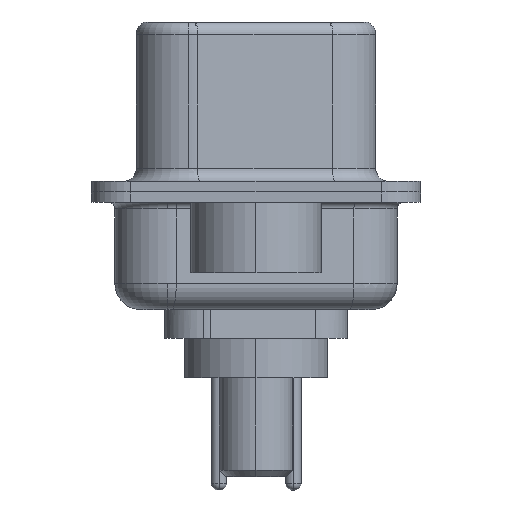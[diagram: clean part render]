
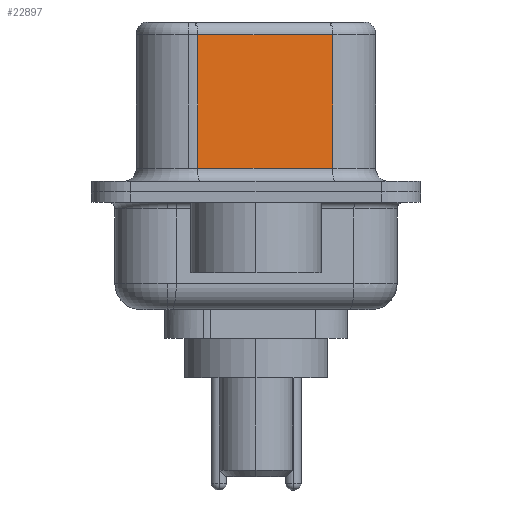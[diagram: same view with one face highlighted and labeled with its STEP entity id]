
A CAD part, left-side view. The second image highlights one B-rep face of the part: STEP entity #22897.
In plain terms, the highlighted planar face has unit normal (-0.985, -0.174, 0).
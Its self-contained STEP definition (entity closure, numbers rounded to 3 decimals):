
#64 = VERTEX_POINT ( 'NONE', #10627 ) ;
#67 = EDGE_CURVE ( 'NONE', #1462, #18568, #2267, .T. ) ;
#1438 = ORIENTED_EDGE ( 'NONE', *, *, #24610, .T. ) ;
#1462 = VERTEX_POINT ( 'NONE', #10594 ) ;
#1481 = CARTESIAN_POINT ( 'NONE',  ( 4.58, -2.927, 6.52 ) ) ;
#2267 = LINE ( 'NONE', #23802, #22901 ) ;
#2606 = VECTOR ( 'NONE', #9799, 1000. ) ;
#3443 = DIRECTION ( 'NONE',  ( 0.985, 0.174, 0. ) ) ;
#3706 = VERTEX_POINT ( 'NONE', #5893 ) ;
#5893 = CARTESIAN_POINT ( 'NONE',  ( 3.67, 2.233, 0.9 ) ) ;
#5898 = LINE ( 'NONE', #21423, #21189 ) ;
#6549 = FACE_OUTER_BOUND ( 'NONE', #18760, .T. ) ;
#6637 = ORIENTED_EDGE ( 'NONE', *, *, #21336, .F. ) ;
#7512 = DIRECTION ( 'NONE',  ( 0., 0., -1. ) ) ;
#9799 = DIRECTION ( 'NONE',  ( 0.174, -0.985, 0. ) ) ;
#10406 = VECTOR ( 'NONE', #7512, 1000. ) ;
#10594 = CARTESIAN_POINT ( 'NONE',  ( 4.58, -2.927, 6.02 ) ) ;
#10627 = CARTESIAN_POINT ( 'NONE',  ( 4.58, -2.927, 0.9 ) ) ;
#13181 = LINE ( 'NONE', #25860, #2606 ) ;
#13431 = CARTESIAN_POINT ( 'NONE',  ( 4.58, -2.927, 6.52 ) ) ;
#15373 = PLANE ( 'NONE',  #18116 ) ;
#16191 = ORIENTED_EDGE ( 'NONE', *, *, #67, .T. ) ;
#17407 = DIRECTION ( 'NONE',  ( -0.174, 0.985, 0. ) ) ;
#17486 = DIRECTION ( 'NONE',  ( 0., 0., -1. ) ) ;
#18116 = AXIS2_PLACEMENT_3D ( 'NONE', #1481, #3443, #17407 ) ;
#18568 = VERTEX_POINT ( 'NONE', #24585 ) ;
#18760 = EDGE_LOOP ( 'NONE', ( #6637, #16191, #1438, #21750 ) ) ;
#21189 = VECTOR ( 'NONE', #17486, 1000. ) ;
#21336 = EDGE_CURVE ( 'NONE', #1462, #64, #21666, .T. ) ;
#21423 = CARTESIAN_POINT ( 'NONE',  ( 3.67, 2.233, 6.52 ) ) ;
#21435 = EDGE_CURVE ( 'NONE', #3706, #64, #13181, .T. ) ;
#21666 = LINE ( 'NONE', #13431, #10406 ) ;
#21750 = ORIENTED_EDGE ( 'NONE', *, *, #21435, .T. ) ;
#22897 = ADVANCED_FACE ( 'NONE', ( #6549 ), #15373, .F. ) ;
#22901 = VECTOR ( 'NONE', #25074, 1000. ) ;
#23802 = CARTESIAN_POINT ( 'NONE',  ( 4.58, -2.927, 6.02 ) ) ;
#24585 = CARTESIAN_POINT ( 'NONE',  ( 3.67, 2.233, 6.02 ) ) ;
#24610 = EDGE_CURVE ( 'NONE', #18568, #3706, #5898, .T. ) ;
#25074 = DIRECTION ( 'NONE',  ( -0.174, 0.985, 0. ) ) ;
#25860 = CARTESIAN_POINT ( 'NONE',  ( 4.58, -2.927, 0.9 ) ) ;
